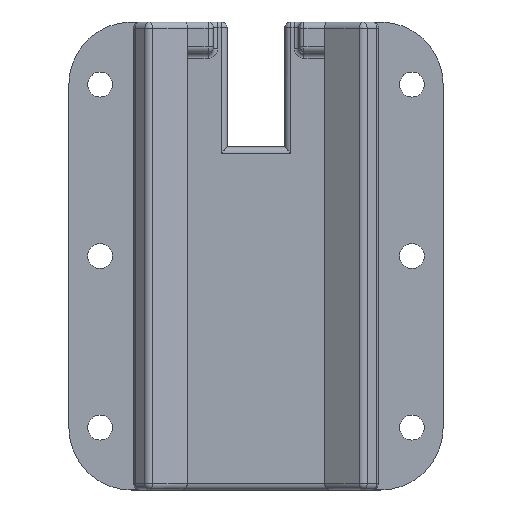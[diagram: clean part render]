
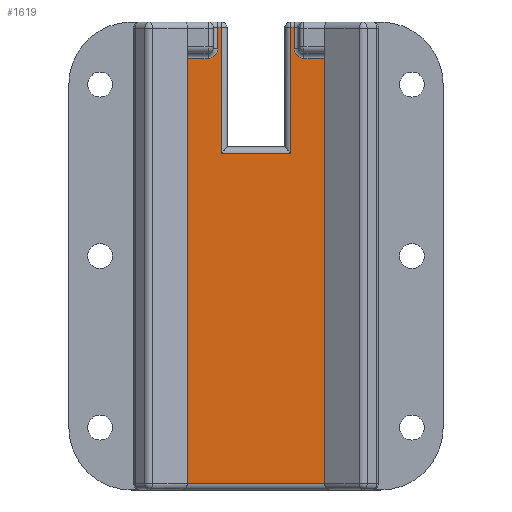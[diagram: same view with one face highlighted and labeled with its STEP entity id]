
A CAD part, top view. The second image highlights one B-rep face of the part: STEP entity #1619.
In plain terms, the highlighted planar face has unit normal (0, 0, 1).
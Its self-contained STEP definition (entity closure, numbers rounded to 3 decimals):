
#68=PLANE('',#1763);
#115=FACE_OUTER_BOUND('',#221,.T.);
#221=EDGE_LOOP('',(#1123,#1124,#1125,#1126,#1127,#1128,#1129,#1130,#1131,
#1132,#1133,#1134,#1135,#1136));
#323=LINE('',#2500,#455);
#324=LINE('',#2585,#456);
#326=LINE('',#2588,#458);
#336=LINE('',#2641,#468);
#338=LINE('',#2647,#470);
#339=LINE('',#2649,#471);
#340=LINE('',#2651,#472);
#341=LINE('',#2653,#473);
#342=LINE('',#2657,#474);
#343=LINE('',#2659,#475);
#344=LINE('',#2661,#476);
#345=LINE('',#2662,#477);
#455=VECTOR('',#1966,10.);
#456=VECTOR('',#1981,10.);
#458=VECTOR('',#1985,10.);
#468=VECTOR('',#2023,1000.);
#470=VECTOR('',#2029,1000.);
#471=VECTOR('',#2030,1000.);
#472=VECTOR('',#2031,1000.);
#473=VECTOR('',#2032,10.);
#474=VECTOR('',#2035,10.);
#475=VECTOR('',#2036,10.);
#476=VECTOR('',#2037,1000.);
#477=VECTOR('',#2038,1000.);
#595=CIRCLE('',#1743,2.);
#607=CIRCLE('',#1764,2.);
#680=VERTEX_POINT('',#2487);
#684=VERTEX_POINT('',#2496);
#689=VERTEX_POINT('',#2576);
#690=VERTEX_POINT('',#2578);
#691=VERTEX_POINT('',#2582);
#703=VERTEX_POINT('',#2640);
#705=VERTEX_POINT('',#2646);
#706=VERTEX_POINT('',#2648);
#707=VERTEX_POINT('',#2650);
#708=VERTEX_POINT('',#2652);
#709=VERTEX_POINT('',#2654);
#710=VERTEX_POINT('',#2656);
#711=VERTEX_POINT('',#2658);
#712=VERTEX_POINT('',#2660);
#830=EDGE_CURVE('',#680,#684,#323,.T.);
#835=EDGE_CURVE('',#689,#690,#595,.T.);
#838=EDGE_CURVE('',#691,#689,#324,.T.);
#840=EDGE_CURVE('',#690,#680,#326,.T.);
#859=EDGE_CURVE('',#703,#684,#336,.T.);
#862=EDGE_CURVE('',#705,#691,#338,.T.);
#863=EDGE_CURVE('',#705,#706,#339,.T.);
#864=EDGE_CURVE('',#706,#707,#340,.T.);
#865=EDGE_CURVE('',#708,#707,#341,.T.);
#866=EDGE_CURVE('',#709,#708,#607,.T.);
#867=EDGE_CURVE('',#710,#709,#342,.T.);
#868=EDGE_CURVE('',#711,#710,#343,.T.);
#869=EDGE_CURVE('',#711,#712,#344,.T.);
#870=EDGE_CURVE('',#712,#703,#345,.T.);
#1123=ORIENTED_EDGE('',*,*,#830,.F.);
#1124=ORIENTED_EDGE('',*,*,#840,.F.);
#1125=ORIENTED_EDGE('',*,*,#835,.F.);
#1126=ORIENTED_EDGE('',*,*,#838,.F.);
#1127=ORIENTED_EDGE('',*,*,#862,.F.);
#1128=ORIENTED_EDGE('',*,*,#863,.T.);
#1129=ORIENTED_EDGE('',*,*,#864,.T.);
#1130=ORIENTED_EDGE('',*,*,#865,.F.);
#1131=ORIENTED_EDGE('',*,*,#866,.F.);
#1132=ORIENTED_EDGE('',*,*,#867,.F.);
#1133=ORIENTED_EDGE('',*,*,#868,.F.);
#1134=ORIENTED_EDGE('',*,*,#869,.T.);
#1135=ORIENTED_EDGE('',*,*,#870,.T.);
#1136=ORIENTED_EDGE('',*,*,#859,.T.);
#1619=ADVANCED_FACE('',(#115),#68,.F.);
#1743=AXIS2_PLACEMENT_3D('',#2579,#1973,#1974);
#1763=AXIS2_PLACEMENT_3D('',#2645,#2027,#2028);
#1764=AXIS2_PLACEMENT_3D('',#2655,#2033,#2034);
#1966=DIRECTION('',(1.,0.,0.));
#1973=DIRECTION('center_axis',(0.,0.,1.));
#1974=DIRECTION('ref_axis',(0.707,-0.707,0.));
#1981=DIRECTION('',(1.,0.,0.));
#1985=DIRECTION('',(0.,1.,0.));
#2023=DIRECTION('',(0.,1.,0.));
#2027=DIRECTION('center_axis',(0.,0.,-1.));
#2028=DIRECTION('ref_axis',(0.,1.,0.));
#2029=DIRECTION('',(0.,1.,0.));
#2030=DIRECTION('',(1.,0.,0.));
#2031=DIRECTION('',(0.,1.,0.));
#2032=DIRECTION('',(1.,0.,0.));
#2033=DIRECTION('center_axis',(0.,0.,1.));
#2034=DIRECTION('ref_axis',(-0.707,-0.707,0.));
#2035=DIRECTION('',(0.,-1.,0.));
#2036=DIRECTION('',(1.,0.,0.));
#2037=DIRECTION('',(0.,-1.,0.));
#2038=DIRECTION('',(-1.,0.,0.));
#2487=CARTESIAN_POINT('',(-7.75,-11.16,10.16));
#2496=CARTESIAN_POINT('',(-7.112,-11.16,10.16));
#2500=CARTESIAN_POINT('',(0.,-11.16,10.16));
#2576=CARTESIAN_POINT('',(-9.75,-17.51,10.16));
#2578=CARTESIAN_POINT('',(-7.75,-15.51,10.16));
#2579=CARTESIAN_POINT('Origin',(-9.75,-15.51,10.16));
#2582=CARTESIAN_POINT('',(-13.97,-17.51,10.16));
#2585=CARTESIAN_POINT('',(-6.223,-17.51,10.16));
#2588=CARTESIAN_POINT('',(-7.75,-57.785,10.16));
#2640=CARTESIAN_POINT('',(-7.112,-36.83,10.16));
#2641=CARTESIAN_POINT('',(-7.112,-105.41,10.16));
#2645=CARTESIAN_POINT('Origin',(0.,-105.41,10.16));
#2646=CARTESIAN_POINT('',(-13.97,-104.14,10.16));
#2647=CARTESIAN_POINT('',(-13.97,-122.863,10.16));
#2648=CARTESIAN_POINT('',(13.97,-104.14,10.16));
#2649=CARTESIAN_POINT('',(13.97,-104.14,10.16));
#2650=CARTESIAN_POINT('',(13.97,-17.51,10.16));
#2651=CARTESIAN_POINT('',(13.97,-122.863,10.16));
#2652=CARTESIAN_POINT('',(9.75,-17.51,10.16));
#2653=CARTESIAN_POINT('',(6.223,-17.51,10.16));
#2654=CARTESIAN_POINT('',(7.75,-15.51,10.16));
#2655=CARTESIAN_POINT('Origin',(9.75,-15.51,10.16));
#2656=CARTESIAN_POINT('',(7.75,-11.16,10.16));
#2657=CARTESIAN_POINT('',(7.75,-57.785,10.16));
#2658=CARTESIAN_POINT('',(7.112,-11.16,10.16));
#2659=CARTESIAN_POINT('',(0.,-11.16,10.16));
#2660=CARTESIAN_POINT('',(7.112,-36.83,10.16));
#2661=CARTESIAN_POINT('',(7.112,-105.41,10.16));
#2662=CARTESIAN_POINT('',(0.,-36.83,10.16));
